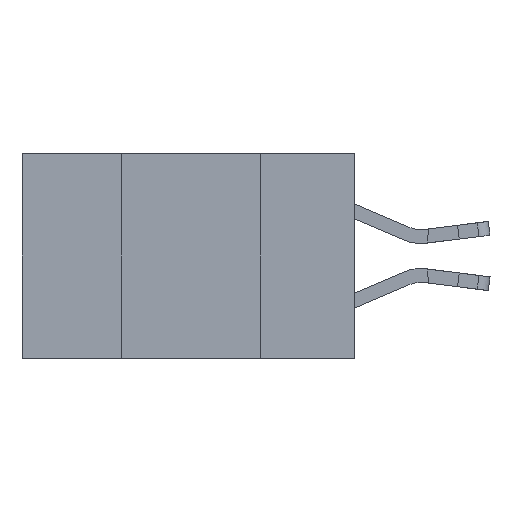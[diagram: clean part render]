
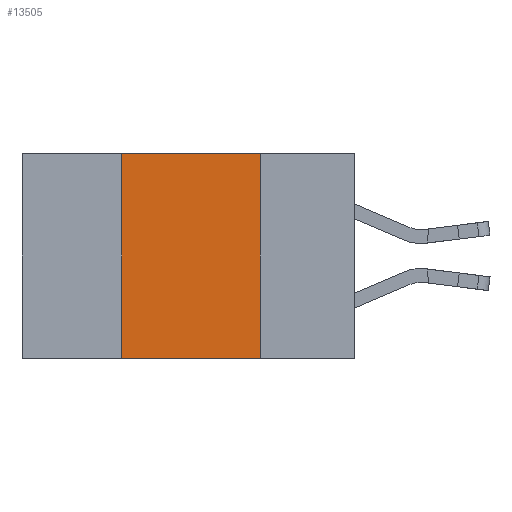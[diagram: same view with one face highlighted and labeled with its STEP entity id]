
A CAD part, left-side view. The second image highlights one B-rep face of the part: STEP entity #13505.
In plain terms, the highlighted planar face has unit normal (-1, 0, 0).
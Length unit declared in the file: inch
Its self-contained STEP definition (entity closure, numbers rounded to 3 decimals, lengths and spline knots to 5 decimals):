
#1156 = AXIS2_PLACEMENT_3D ( 'NONE', #10918, #6237, #17073 ) ;
#1417 = PLANE ( 'NONE',  #1156 ) ;
#3065 = VECTOR ( 'NONE', #13744, 39.37008 ) ;
#3135 = DIRECTION ( 'NONE',  ( 0., -1., 0. ) ) ;
#3539 = ORIENTED_EDGE ( 'NONE', *, *, #10269, .F. ) ;
#3909 = ORIENTED_EDGE ( 'NONE', *, *, #16294, .F. ) ;
#4395 = VERTEX_POINT ( 'NONE', #16097 ) ;
#4904 = EDGE_LOOP ( 'NONE', ( #3539, #3909, #5862, #6726 ) ) ;
#5862 = ORIENTED_EDGE ( 'NONE', *, *, #9212, .F. ) ;
#6237 = DIRECTION ( 'NONE',  ( 1., 0., 0. ) ) ;
#6726 = ORIENTED_EDGE ( 'NONE', *, *, #8136, .T. ) ;
#7024 = LINE ( 'NONE', #18575, #15308 ) ;
#8079 = LINE ( 'NONE', #18518, #11743 ) ;
#8136 = EDGE_CURVE ( 'NONE', #18709, #14765, #16347, .T. ) ;
#9212 = EDGE_CURVE ( 'NONE', #18709, #4395, #8079, .T. ) ;
#10269 = EDGE_CURVE ( 'NONE', #13627, #14765, #11444, .T. ) ;
#10855 = FACE_OUTER_BOUND ( 'NONE', #4904, .T. ) ;
#10918 = CARTESIAN_POINT ( 'NONE',  ( 0., 0.6, 0. ) ) ;
#11444 = LINE ( 'NONE', #18234, #3065 ) ;
#11743 = VECTOR ( 'NONE', #12469, 39.37008 ) ;
#11800 = VECTOR ( 'NONE', #16831, 39.37008 ) ;
#12469 = DIRECTION ( 'NONE',  ( 0., 0., 1. ) ) ;
#12622 = CARTESIAN_POINT ( 'NONE',  ( 0., 0.17, 0. ) ) ;
#13505 = ADVANCED_FACE ( 'NONE', ( #10855 ), #1417, .F. ) ;
#13627 = VERTEX_POINT ( 'NONE', #12622 ) ;
#13744 = DIRECTION ( 'NONE',  ( 0., 0., -1. ) ) ;
#14765 = VERTEX_POINT ( 'NONE', #19776 ) ;
#15308 = VECTOR ( 'NONE', #3135, 39.37008 ) ;
#15329 = CARTESIAN_POINT ( 'NONE',  ( 0., 0.6, -0.37 ) ) ;
#15922 = CARTESIAN_POINT ( 'NONE',  ( 0., 0.42, -0.37 ) ) ;
#16097 = CARTESIAN_POINT ( 'NONE',  ( 0., 0.42, 0. ) ) ;
#16294 = EDGE_CURVE ( 'NONE', #4395, #13627, #7024, .T. ) ;
#16347 = LINE ( 'NONE', #15329, #11800 ) ;
#16831 = DIRECTION ( 'NONE',  ( 0., -1., 0. ) ) ;
#17073 = DIRECTION ( 'NONE',  ( 0., 0., -1. ) ) ;
#18234 = CARTESIAN_POINT ( 'NONE',  ( 0., 0.17, 0. ) ) ;
#18518 = CARTESIAN_POINT ( 'NONE',  ( 0., 0.42, 0. ) ) ;
#18575 = CARTESIAN_POINT ( 'NONE',  ( 0., 0.6, 0. ) ) ;
#18709 = VERTEX_POINT ( 'NONE', #15922 ) ;
#19776 = CARTESIAN_POINT ( 'NONE',  ( 0., 0.17, -0.37 ) ) ;
